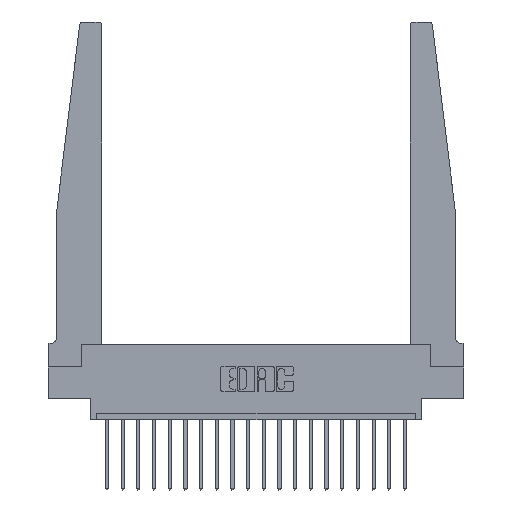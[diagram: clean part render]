
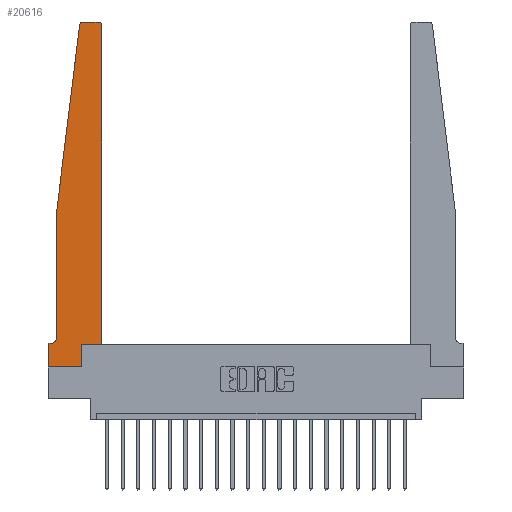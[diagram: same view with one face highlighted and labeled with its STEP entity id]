
A CAD part, top view. The second image highlights one B-rep face of the part: STEP entity #20616.
In plain terms, the highlighted planar face has unit normal (0, 0, 1).
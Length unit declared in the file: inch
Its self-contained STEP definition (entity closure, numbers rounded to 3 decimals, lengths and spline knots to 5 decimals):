
#3 = CARTESIAN_POINT ( 'NONE',  ( 0.25, 2.75, 0.37 ) ) ;
#43 = ORIENTED_EDGE ( 'NONE', *, *, #12584, .T. ) ;
#102 = LINE ( 'NONE', #12903, #19973 ) ;
#295 = AXIS2_PLACEMENT_3D ( 'NONE', #10323, #2045, #5305 ) ;
#389 = EDGE_CURVE ( 'NONE', #15073, #8148, #11171, .T. ) ;
#732 = CARTESIAN_POINT ( 'NONE',  ( 0.395, 2.75, 0.37 ) ) ;
#1275 = DIRECTION ( 'NONE',  ( 1., 0., 0. ) ) ;
#1357 = CARTESIAN_POINT ( 'NONE',  ( 0.27653, 2.72, 0.37 ) ) ;
#1437 = EDGE_CURVE ( 'NONE', #10562, #9060, #4004, .T. ) ;
#1575 = EDGE_CURVE ( 'NONE', #17279, #4591, #9388, .T. ) ;
#1717 = DIRECTION ( 'NONE',  ( -0.122, -0.992, 0. ) ) ;
#1837 = CARTESIAN_POINT ( 'NONE',  ( 0.065, 0.1875, 0.37 ) ) ;
#1980 = CARTESIAN_POINT ( 'NONE',  ( 0., 0., 0.37 ) ) ;
#2045 = DIRECTION ( 'NONE',  ( 0., 0., 1. ) ) ;
#2151 = FACE_OUTER_BOUND ( 'NONE', #6215, .T. ) ;
#2239 = CARTESIAN_POINT ( 'NONE',  ( 0.395, 2.72, 0.37 ) ) ;
#2862 = EDGE_CURVE ( 'NONE', #13010, #10562, #102, .T. ) ;
#3196 = LINE ( 'NONE', #10838, #5314 ) ;
#3886 = EDGE_CURVE ( 'NONE', #9060, #10748, #5941, .T. ) ;
#4003 = CARTESIAN_POINT ( 'NONE',  ( 0., 0., 0.37 ) ) ;
#4004 = LINE ( 'NONE', #18567, #10347 ) ;
#4127 = ORIENTED_EDGE ( 'NONE', *, *, #20406, .T. ) ;
#4129 = DIRECTION ( 'NONE',  ( 1., 0., 0. ) ) ;
#4221 = DIRECTION ( 'NONE',  ( 0., 1., 0. ) ) ;
#4322 = CARTESIAN_POINT ( 'NONE',  ( 0.015, 0.1875, 0.37 ) ) ;
#4368 = ORIENTED_EDGE ( 'NONE', *, *, #3886, .T. ) ;
#4488 = VERTEX_POINT ( 'NONE', #14353 ) ;
#4591 = VERTEX_POINT ( 'NONE', #17031 ) ;
#5007 = LINE ( 'NONE', #14531, #11349 ) ;
#5244 = LINE ( 'NONE', #1980, #10131 ) ;
#5305 = DIRECTION ( 'NONE',  ( 1., 0., 0. ) ) ;
#5314 = VECTOR ( 'NONE', #17228, 39.37008 ) ;
#5787 = ORIENTED_EDGE ( 'NONE', *, *, #389, .T. ) ;
#5941 = CIRCLE ( 'NONE', #17643, 0.03 ) ;
#6215 = EDGE_LOOP ( 'NONE', ( #9745, #18664, #43, #8783, #5787, #4127, #19133, #18271, #13285, #19101, #8161, #4368 ) ) ;
#6384 = CARTESIAN_POINT ( 'NONE',  ( 0.015, 0.2375, 0.37 ) ) ;
#6465 = DIRECTION ( 'NONE',  ( -1., 0., 0. ) ) ;
#6672 = EDGE_CURVE ( 'NONE', #17992, #10649, #15110, .T. ) ;
#7706 = AXIS2_PLACEMENT_3D ( 'NONE', #1357, #12583, #1275 ) ;
#8108 = LINE ( 'NONE', #12927, #12537 ) ;
#8148 = VERTEX_POINT ( 'NONE', #4322 ) ;
#8161 = ORIENTED_EDGE ( 'NONE', *, *, #1437, .T. ) ;
#8231 = LINE ( 'NONE', #1837, #20706 ) ;
#8244 = EDGE_CURVE ( 'NONE', #4488, #17992, #5244, .T. ) ;
#8284 = CARTESIAN_POINT ( 'NONE',  ( 0.2605, 0.18, 0.37 ) ) ;
#8783 = ORIENTED_EDGE ( 'NONE', *, *, #18572, .T. ) ;
#9060 = VERTEX_POINT ( 'NONE', #9876 ) ;
#9388 = CIRCLE ( 'NONE', #7706, 0.03 ) ;
#9558 = LINE ( 'NONE', #3, #17539 ) ;
#9745 = ORIENTED_EDGE ( 'NONE', *, *, #11803, .T. ) ;
#9876 = CARTESIAN_POINT ( 'NONE',  ( 0.425, 2.72, 0.37 ) ) ;
#9955 = CARTESIAN_POINT ( 'NONE',  ( 0.2605, 0., 0.37 ) ) ;
#10131 = VECTOR ( 'NONE', #18018, 39.37008 ) ;
#10323 = CARTESIAN_POINT ( 'NONE',  ( 0., 0.1875, 0.37 ) ) ;
#10347 = VECTOR ( 'NONE', #4221, 39.37008 ) ;
#10562 = VERTEX_POINT ( 'NONE', #17821 ) ;
#10649 = VERTEX_POINT ( 'NONE', #9955 ) ;
#10748 = VERTEX_POINT ( 'NONE', #732 ) ;
#10838 = CARTESIAN_POINT ( 'NONE',  ( 0.065, 1.25, 0.37 ) ) ;
#11171 = CIRCLE ( 'NONE', #19211, 0.05 ) ;
#11218 = DIRECTION ( 'NONE',  ( -1., 0., 0. ) ) ;
#11349 = VECTOR ( 'NONE', #15691, 39.37008 ) ;
#11803 = EDGE_CURVE ( 'NONE', #10748, #17279, #9558, .T. ) ;
#12537 = VECTOR ( 'NONE', #1717, 39.37008 ) ;
#12583 = DIRECTION ( 'NONE',  ( 0., 0., 1. ) ) ;
#12584 = EDGE_CURVE ( 'NONE', #4591, #19844, #8108, .T. ) ;
#12765 = DIRECTION ( 'NONE',  ( -1., 0., 0. ) ) ;
#12903 = CARTESIAN_POINT ( 'NONE',  ( 0.425, 0.18, 0.37 ) ) ;
#12927 = CARTESIAN_POINT ( 'NONE',  ( 0.065, 1.25, 0.37 ) ) ;
#13010 = VERTEX_POINT ( 'NONE', #8284 ) ;
#13285 = ORIENTED_EDGE ( 'NONE', *, *, #18031, .T. ) ;
#13517 = CARTESIAN_POINT ( 'NONE',  ( 0.065, 0.2375, 0.37 ) ) ;
#13535 = DIRECTION ( 'NONE',  ( 1., 0., 0. ) ) ;
#14353 = CARTESIAN_POINT ( 'NONE',  ( 0., 0.1875, 0.37 ) ) ;
#14531 = CARTESIAN_POINT ( 'NONE',  ( 0.2605, 0.18, 0.37 ) ) ;
#15073 = VERTEX_POINT ( 'NONE', #13517 ) ;
#15110 = LINE ( 'NONE', #4003, #19809 ) ;
#15691 = DIRECTION ( 'NONE',  ( 0., 1., 0. ) ) ;
#17031 = CARTESIAN_POINT ( 'NONE',  ( 0.24675, 2.72367, 0.37 ) ) ;
#17228 = DIRECTION ( 'NONE',  ( 0., -1., 0. ) ) ;
#17279 = VERTEX_POINT ( 'NONE', #19221 ) ;
#17539 = VECTOR ( 'NONE', #11218, 39.37008 ) ;
#17643 = AXIS2_PLACEMENT_3D ( 'NONE', #2239, #19631, #4129 ) ;
#17793 = DIRECTION ( 'NONE',  ( 0., 0., -1. ) ) ;
#17821 = CARTESIAN_POINT ( 'NONE',  ( 0.425, 0.18, 0.37 ) ) ;
#17992 = VERTEX_POINT ( 'NONE', #19251 ) ;
#18018 = DIRECTION ( 'NONE',  ( 0., -1., 0. ) ) ;
#18031 = EDGE_CURVE ( 'NONE', #10649, #13010, #5007, .T. ) ;
#18271 = ORIENTED_EDGE ( 'NONE', *, *, #6672, .T. ) ;
#18567 = CARTESIAN_POINT ( 'NONE',  ( 0.425, 0.18, 0.37 ) ) ;
#18572 = EDGE_CURVE ( 'NONE', #19844, #15073, #3196, .T. ) ;
#18664 = ORIENTED_EDGE ( 'NONE', *, *, #1575, .T. ) ;
#18855 = CARTESIAN_POINT ( 'NONE',  ( 0.065, 1.25, 0.37 ) ) ;
#19101 = ORIENTED_EDGE ( 'NONE', *, *, #2862, .T. ) ;
#19133 = ORIENTED_EDGE ( 'NONE', *, *, #8244, .T. ) ;
#19211 = AXIS2_PLACEMENT_3D ( 'NONE', #6384, #17793, #12765 ) ;
#19221 = CARTESIAN_POINT ( 'NONE',  ( 0.27653, 2.75, 0.37 ) ) ;
#19251 = CARTESIAN_POINT ( 'NONE',  ( 0., 0., 0.37 ) ) ;
#19631 = DIRECTION ( 'NONE',  ( 0., 0., 1. ) ) ;
#19647 = PLANE ( 'NONE',  #295 ) ;
#19809 = VECTOR ( 'NONE', #13535, 39.37008 ) ;
#19844 = VERTEX_POINT ( 'NONE', #18855 ) ;
#19973 = VECTOR ( 'NONE', #20651, 39.37008 ) ;
#20406 = EDGE_CURVE ( 'NONE', #8148, #4488, #8231, .T. ) ;
#20616 = ADVANCED_FACE ( 'NONE', ( #2151 ), #19647, .T. ) ;
#20651 = DIRECTION ( 'NONE',  ( 1., 0., 0. ) ) ;
#20706 = VECTOR ( 'NONE', #6465, 39.37008 ) ;
